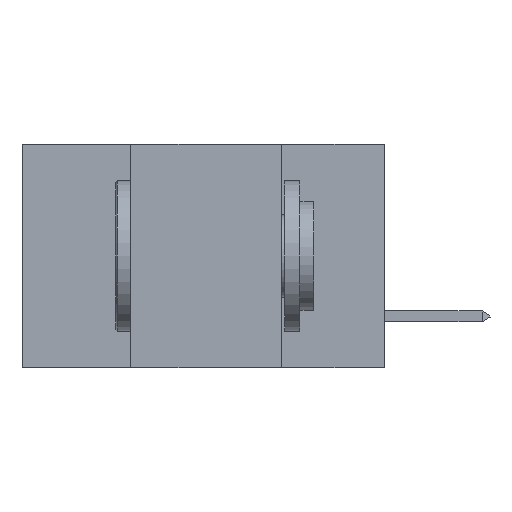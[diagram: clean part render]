
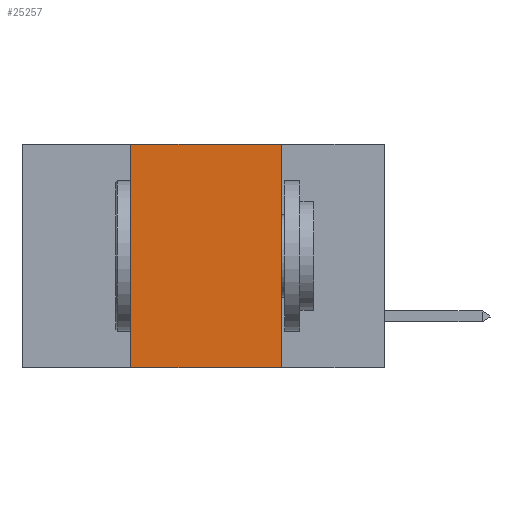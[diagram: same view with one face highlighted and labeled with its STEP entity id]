
A CAD part, left-side view. The second image highlights one B-rep face of the part: STEP entity #25257.
In plain terms, the highlighted planar face has unit normal (-1, 0, 0).
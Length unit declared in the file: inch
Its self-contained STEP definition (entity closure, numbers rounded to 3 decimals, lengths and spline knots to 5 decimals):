
#1841 = EDGE_CURVE ( 'NONE', #27961, #5959, #10619, .T. ) ;
#2900 = AXIS2_PLACEMENT_3D ( 'NONE', #43036, #11474, #42894 ) ;
#3748 = DIRECTION ( 'NONE',  ( 0., -1., 0. ) ) ;
#3970 = LINE ( 'NONE', #17126, #44565 ) ;
#4384 = CARTESIAN_POINT ( 'NONE',  ( 0., 0.17, -0.37 ) ) ;
#4403 = CARTESIAN_POINT ( 'NONE',  ( 0., 0.17, 0. ) ) ;
#4941 = VERTEX_POINT ( 'NONE', #4403 ) ;
#5959 = VERTEX_POINT ( 'NONE', #4384 ) ;
#9046 = LINE ( 'NONE', #40123, #45776 ) ;
#10619 = LINE ( 'NONE', #28361, #34506 ) ;
#11474 = DIRECTION ( 'NONE',  ( 1., 0., 0. ) ) ;
#12310 = LINE ( 'NONE', #43076, #33968 ) ;
#15230 = CARTESIAN_POINT ( 'NONE',  ( 0., 0.42, -0.37 ) ) ;
#17126 = CARTESIAN_POINT ( 'NONE',  ( 0., 0.42, 0. ) ) ;
#17588 = DIRECTION ( 'NONE',  ( 0., 0., 1. ) ) ;
#19125 = DIRECTION ( 'NONE',  ( 0., 0., -1. ) ) ;
#19229 = ORIENTED_EDGE ( 'NONE', *, *, #26393, .F. ) ;
#20288 = ORIENTED_EDGE ( 'NONE', *, *, #26467, .F. ) ;
#21728 = PLANE ( 'NONE',  #2900 ) ;
#25257 = ADVANCED_FACE ( 'NONE', ( #41944 ), #21728, .F. ) ;
#25372 = VERTEX_POINT ( 'NONE', #33026 ) ;
#26393 = EDGE_CURVE ( 'NONE', #27961, #25372, #3970, .T. ) ;
#26467 = EDGE_CURVE ( 'NONE', #25372, #4941, #12310, .T. ) ;
#27961 = VERTEX_POINT ( 'NONE', #15230 ) ;
#28361 = CARTESIAN_POINT ( 'NONE',  ( 0., 0.6, -0.37 ) ) ;
#29961 = EDGE_LOOP ( 'NONE', ( #45111, #20288, #19229, #44210 ) ) ;
#32955 = EDGE_CURVE ( 'NONE', #4941, #5959, #9046, .T. ) ;
#33026 = CARTESIAN_POINT ( 'NONE',  ( 0., 0.42, 0. ) ) ;
#33968 = VECTOR ( 'NONE', #3748, 39.37008 ) ;
#34506 = VECTOR ( 'NONE', #39084, 39.37008 ) ;
#39084 = DIRECTION ( 'NONE',  ( 0., -1., 0. ) ) ;
#40123 = CARTESIAN_POINT ( 'NONE',  ( 0., 0.17, 0. ) ) ;
#41944 = FACE_OUTER_BOUND ( 'NONE', #29961, .T. ) ;
#42894 = DIRECTION ( 'NONE',  ( 0., 0., -1. ) ) ;
#43036 = CARTESIAN_POINT ( 'NONE',  ( 0., 0.6, 0. ) ) ;
#43076 = CARTESIAN_POINT ( 'NONE',  ( 0., 0.6, 0. ) ) ;
#44210 = ORIENTED_EDGE ( 'NONE', *, *, #1841, .T. ) ;
#44565 = VECTOR ( 'NONE', #17588, 39.37008 ) ;
#45111 = ORIENTED_EDGE ( 'NONE', *, *, #32955, .F. ) ;
#45776 = VECTOR ( 'NONE', #19125, 39.37008 ) ;
